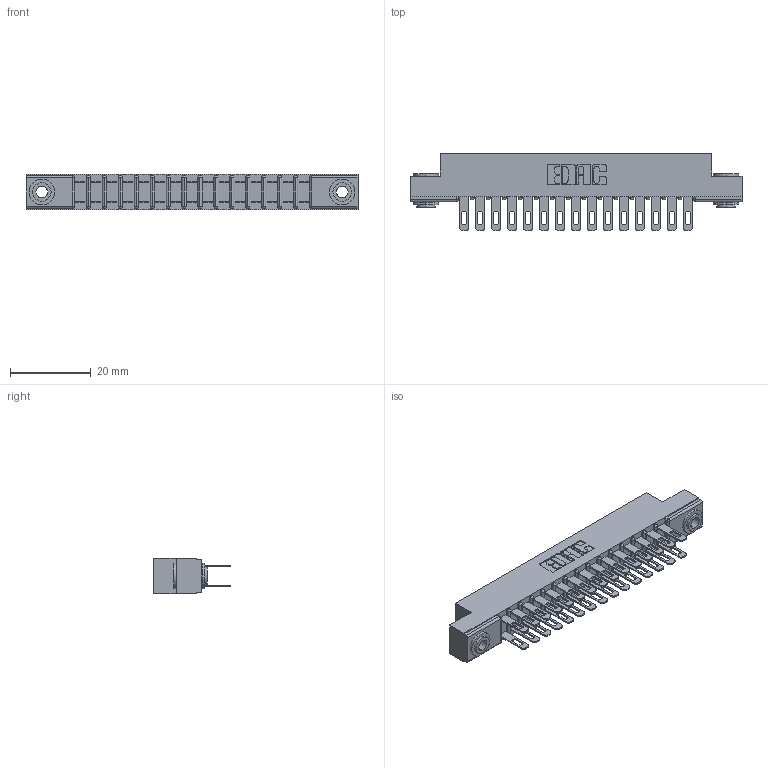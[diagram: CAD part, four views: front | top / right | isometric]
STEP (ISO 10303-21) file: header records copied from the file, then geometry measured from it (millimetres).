
FILE_DESCRIPTION (( 'STEP AP203' ), '1' );
FILE_NAME ('307-030-400-203.STEP', '2020-09-29T08:53:57', ( '' ), ( '' ), 'SwSTEP 2.0', 'SolidWorks 2020', '' );
FILE_SCHEMA (( 'CONFIG_CONTROL_DESIGN' ));
Length unit declared in the file: inch
Products named in the file (4): 307-030-400-203; 345-250-002_345-250-002-102; 307 Part_.156 Dia Mounting Holes; 307-290-001_500
Assembly tree (33 placements, depth 2):
  307-030-400-203
    307 Part_.156 Dia Mounting Holes
    307-290-001_500  x30
    345-250-002_345-250-002-102  x2
Bounding box: 82.45 x 19.18 x 8.71 mm (x, y, z)
Volume: 5481 mm3; surface area: 10040 mm2
Topology: 33 solids, 33 shells, 1566 faces, 4335 edges, 2802 vertices
Faces by surface type: plane 994, cylinder 532, sphere 32, cone 8
Entity records: 17707 total; most frequent: CARTESIAN_POINT 2884, DIRECTION 2853, ORIENTED_EDGE 2846, EDGE_CURVE 1423, VECTOR 1071, LINE 1071, VERTEX_POINT 922, AXIS2_PLACEMENT_3D 891
